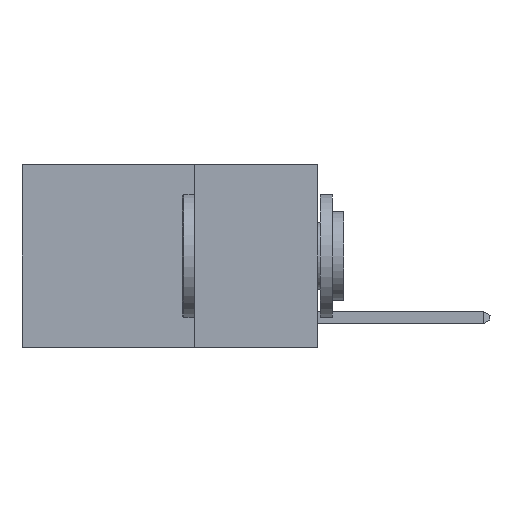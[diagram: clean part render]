
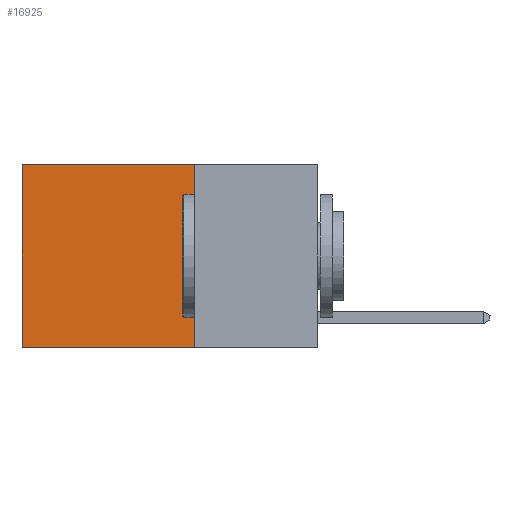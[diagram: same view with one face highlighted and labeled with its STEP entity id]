
A CAD part, left-side view. The second image highlights one B-rep face of the part: STEP entity #16925.
In plain terms, the highlighted planar face has unit normal (-1, 0, 0).
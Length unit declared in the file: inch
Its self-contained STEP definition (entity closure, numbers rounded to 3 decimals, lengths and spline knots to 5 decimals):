
#1182 = LINE ( 'NONE', #9409, #3750 ) ;
#1424 = ORIENTED_EDGE ( 'NONE', *, *, #17721, .F. ) ;
#1835 = VECTOR ( 'NONE', #2831, 39.37008 ) ;
#2831 = DIRECTION ( 'NONE',  ( 0., 1., 0. ) ) ;
#3013 = DIRECTION ( 'NONE',  ( 0., 0., -1. ) ) ;
#3225 = DIRECTION ( 'NONE',  ( 0., 0., -1. ) ) ;
#3750 = VECTOR ( 'NONE', #14723, 39.37008 ) ;
#3833 = ORIENTED_EDGE ( 'NONE', *, *, #6418, .T. ) ;
#3979 = CARTESIAN_POINT ( 'NONE',  ( 0.2625, 0.25, -0.37 ) ) ;
#4502 = EDGE_CURVE ( 'NONE', #5271, #6219, #8080, .T. ) ;
#4807 = ORIENTED_EDGE ( 'NONE', *, *, #15477, .F. ) ;
#4932 = ORIENTED_EDGE ( 'NONE', *, *, #4502, .T. ) ;
#5271 = VERTEX_POINT ( 'NONE', #17347 ) ;
#5795 = LINE ( 'NONE', #7157, #1835 ) ;
#6219 = VERTEX_POINT ( 'NONE', #17541 ) ;
#6418 = EDGE_CURVE ( 'NONE', #14754, #5271, #5795, .T. ) ;
#6627 = CARTESIAN_POINT ( 'NONE',  ( 0.2625, 0.25, 0. ) ) ;
#7157 = CARTESIAN_POINT ( 'NONE',  ( 0.2625, 0.25, 0. ) ) ;
#7176 = CARTESIAN_POINT ( 'NONE',  ( 0.2625, 0.25, 0. ) ) ;
#7480 = CARTESIAN_POINT ( 'NONE',  ( 0.2625, 0.25, 0. ) ) ;
#8080 = LINE ( 'NONE', #17914, #17699 ) ;
#8739 = LINE ( 'NONE', #7480, #10105 ) ;
#9409 = CARTESIAN_POINT ( 'NONE',  ( 0.2625, 0.25, -0.37 ) ) ;
#9802 = EDGE_LOOP ( 'NONE', ( #4932, #1424, #4807, #3833 ) ) ;
#10105 = VECTOR ( 'NONE', #3225, 39.37008 ) ;
#12525 = DIRECTION ( 'NONE',  ( 1., 0., 0. ) ) ;
#12617 = FACE_OUTER_BOUND ( 'NONE', #9802, .T. ) ;
#14723 = DIRECTION ( 'NONE',  ( 0., 1., 0. ) ) ;
#14754 = VERTEX_POINT ( 'NONE', #6627 ) ;
#15477 = EDGE_CURVE ( 'NONE', #14754, #17764, #8739, .T. ) ;
#16781 = AXIS2_PLACEMENT_3D ( 'NONE', #7176, #12525, #3013 ) ;
#16925 = ADVANCED_FACE ( 'NONE', ( #12617 ), #17001, .F. ) ;
#17001 = PLANE ( 'NONE',  #16781 ) ;
#17347 = CARTESIAN_POINT ( 'NONE',  ( 0.2625, 0.6, 0. ) ) ;
#17541 = CARTESIAN_POINT ( 'NONE',  ( 0.2625, 0.6, -0.37 ) ) ;
#17699 = VECTOR ( 'NONE', #17814, 39.37008 ) ;
#17721 = EDGE_CURVE ( 'NONE', #17764, #6219, #1182, .T. ) ;
#17764 = VERTEX_POINT ( 'NONE', #3979 ) ;
#17814 = DIRECTION ( 'NONE',  ( 0., 0., -1. ) ) ;
#17914 = CARTESIAN_POINT ( 'NONE',  ( 0.2625, 0.6, 0. ) ) ;
